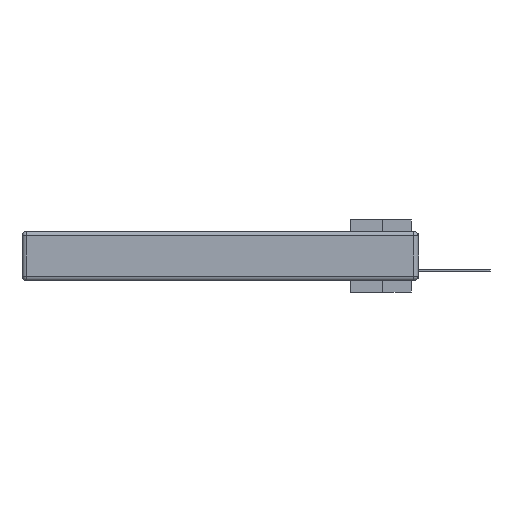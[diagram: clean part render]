
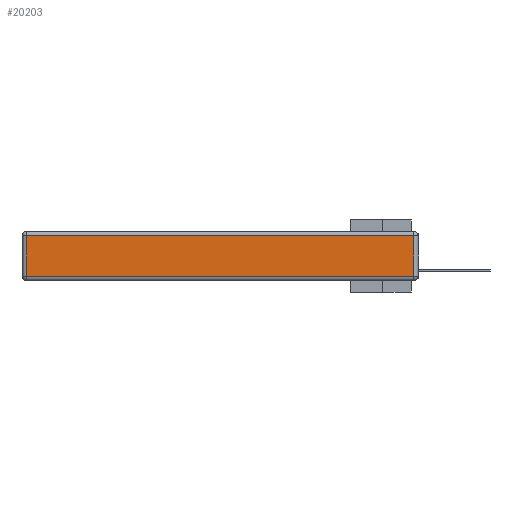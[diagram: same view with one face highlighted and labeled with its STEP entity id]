
A CAD part, left-side view. The second image highlights one B-rep face of the part: STEP entity #20203.
In plain terms, the highlighted planar face has unit normal (-1, 0, 0).
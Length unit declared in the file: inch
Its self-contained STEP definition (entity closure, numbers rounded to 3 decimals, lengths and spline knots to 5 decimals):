
#996 = DIRECTION ( 'NONE',  ( 0., 1., 0. ) ) ;
#1596 = EDGE_CURVE ( 'NONE', #7834, #33946, #12089, .T. ) ;
#1819 = DIRECTION ( 'NONE',  ( 0., 0., 1. ) ) ;
#2403 = DIRECTION ( 'NONE',  ( 0., 0., -1. ) ) ;
#2449 = VERTEX_POINT ( 'NONE', #23764 ) ;
#3210 = EDGE_CURVE ( 'NONE', #12986, #2449, #31952, .T. ) ;
#4769 = LINE ( 'NONE', #33027, #22189 ) ;
#5184 = VECTOR ( 'NONE', #996, 39.37008 ) ;
#5445 = AXIS2_PLACEMENT_3D ( 'NONE', #26847, #27361, #7830 ) ;
#6918 = ORIENTED_EDGE ( 'NONE', *, *, #1596, .T. ) ;
#7830 = DIRECTION ( 'NONE',  ( 0., 0., 1. ) ) ;
#7834 = VERTEX_POINT ( 'NONE', #27393 ) ;
#8216 = EDGE_CURVE ( 'NONE', #33946, #12986, #20710, .T. ) ;
#10679 = ORIENTED_EDGE ( 'NONE', *, *, #3210, .T. ) ;
#11558 = ORIENTED_EDGE ( 'NONE', *, *, #19738, .T. ) ;
#12089 = LINE ( 'NONE', #23486, #34385 ) ;
#12986 = VERTEX_POINT ( 'NONE', #13159 ) ;
#13159 = CARTESIAN_POINT ( 'NONE',  ( 0., 0.03, -0.03 ) ) ;
#13195 = ORIENTED_EDGE ( 'NONE', *, *, #8216, .T. ) ;
#13276 = PLANE ( 'NONE',  #5445 ) ;
#15721 = EDGE_LOOP ( 'NONE', ( #6918, #13195, #10679, #11558 ) ) ;
#16335 = FACE_OUTER_BOUND ( 'NONE', #15721, .T. ) ;
#19738 = EDGE_CURVE ( 'NONE', #2449, #7834, #4769, .T. ) ;
#20203 = ADVANCED_FACE ( 'NONE', ( #16335 ), #13276, .T. ) ;
#20710 = LINE ( 'NONE', #32082, #32950 ) ;
#22189 = VECTOR ( 'NONE', #2403, 39.37008 ) ;
#23143 = DIRECTION ( 'NONE',  ( 0., -1., 0. ) ) ;
#23486 = CARTESIAN_POINT ( 'NONE',  ( 0., 0., -0.313 ) ) ;
#23764 = CARTESIAN_POINT ( 'NONE',  ( 0., 2.72, -0.03 ) ) ;
#26355 = CARTESIAN_POINT ( 'NONE',  ( 0., 2.75, -0.03 ) ) ;
#26847 = CARTESIAN_POINT ( 'NONE',  ( 0., 0., -0.343 ) ) ;
#27361 = DIRECTION ( 'NONE',  ( -1., 0., 0. ) ) ;
#27393 = CARTESIAN_POINT ( 'NONE',  ( 0., 2.72, -0.313 ) ) ;
#31952 = LINE ( 'NONE', #26355, #5184 ) ;
#32082 = CARTESIAN_POINT ( 'NONE',  ( 0., 0.03, -0.343 ) ) ;
#32950 = VECTOR ( 'NONE', #1819, 39.37008 ) ;
#33027 = CARTESIAN_POINT ( 'NONE',  ( 0., 2.72, -0.343 ) ) ;
#33946 = VERTEX_POINT ( 'NONE', #34026 ) ;
#34026 = CARTESIAN_POINT ( 'NONE',  ( 0., 0.03, -0.313 ) ) ;
#34385 = VECTOR ( 'NONE', #23143, 39.37008 ) ;
